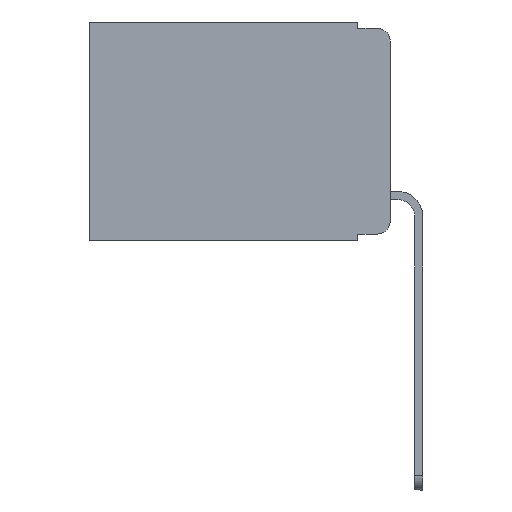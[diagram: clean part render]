
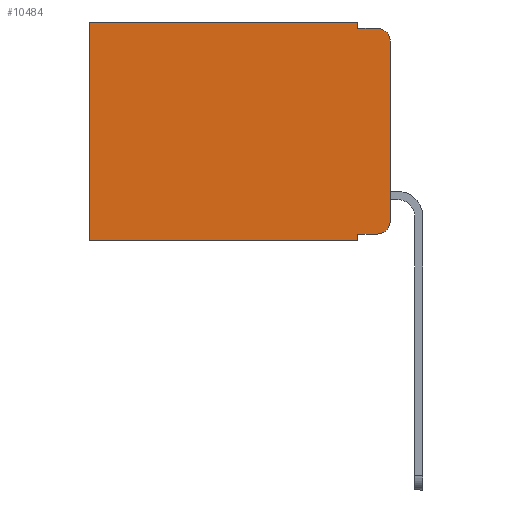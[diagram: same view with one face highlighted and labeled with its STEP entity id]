
A CAD part, left-side view. The second image highlights one B-rep face of the part: STEP entity #10484.
In plain terms, the highlighted planar face has unit normal (-1, 0, 0).
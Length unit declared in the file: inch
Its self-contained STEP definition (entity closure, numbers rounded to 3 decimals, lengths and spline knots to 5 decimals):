
#246 = CARTESIAN_POINT ( 'NONE',  ( 0.298, 0.473, 0. ) ) ;
#336 = VERTEX_POINT ( 'NONE', #1323 ) ;
#412 = DIRECTION ( 'NONE',  ( 0., 1., 0. ) ) ;
#596 = DIRECTION ( 'NONE',  ( 0., 0., -1. ) ) ;
#643 = DIRECTION ( 'NONE',  ( 0., 0., -1. ) ) ;
#776 = CARTESIAN_POINT ( 'NONE',  ( 0.298, 0., -0.343 ) ) ;
#867 = ORIENTED_EDGE ( 'NONE', *, *, #1271, .F. ) ;
#1121 = VERTEX_POINT ( 'NONE', #10203 ) ;
#1159 = ORIENTED_EDGE ( 'NONE', *, *, #6632, .T. ) ;
#1271 = EDGE_CURVE ( 'NONE', #4953, #336, #5555, .T. ) ;
#1323 = CARTESIAN_POINT ( 'NONE',  ( 0.298, 0.02, -0.01 ) ) ;
#1440 = VECTOR ( 'NONE', #6794, 39.37008 ) ;
#1689 = LINE ( 'NONE', #5073, #1440 ) ;
#2042 = EDGE_CURVE ( 'NONE', #4175, #6523, #2232, .T. ) ;
#2195 = LINE ( 'NONE', #9976, #4772 ) ;
#2226 = DIRECTION ( 'NONE',  ( -1., 0., 0. ) ) ;
#2232 = LINE ( 'NONE', #4803, #10056 ) ;
#2279 = EDGE_LOOP ( 'NONE', ( #7759, #1159, #867, #7709, #9970, #9545, #9791, #10288, #2956, #4319 ) ) ;
#2368 = CARTESIAN_POINT ( 'NONE',  ( 0.298, 0., 0. ) ) ;
#2416 = DIRECTION ( 'NONE',  ( 0., 0., -1. ) ) ;
#2614 = CARTESIAN_POINT ( 'NONE',  ( 0.298, 0., -0.03 ) ) ;
#2847 = DIRECTION ( 'NONE',  ( 0., -1., 0. ) ) ;
#2956 = ORIENTED_EDGE ( 'NONE', *, *, #5288, .T. ) ;
#3245 = CARTESIAN_POINT ( 'NONE',  ( 0.298, 0., 0. ) ) ;
#3352 = DIRECTION ( 'NONE',  ( 0., 0., -1. ) ) ;
#3495 = EDGE_CURVE ( 'NONE', #6523, #5057, #2195, .T. ) ;
#3515 = CARTESIAN_POINT ( 'NONE',  ( 0.298, 0.051, -0.333 ) ) ;
#3539 = VERTEX_POINT ( 'NONE', #5753 ) ;
#3548 = CIRCLE ( 'NONE', #7241, 0.02 ) ;
#4175 = VERTEX_POINT ( 'NONE', #5488 ) ;
#4253 = LINE ( 'NONE', #3245, #5478 ) ;
#4319 = ORIENTED_EDGE ( 'NONE', *, *, #6346, .T. ) ;
#4366 = DIRECTION ( 'NONE',  ( 0., -1., 0. ) ) ;
#4491 = VECTOR ( 'NONE', #8370, 39.37008 ) ;
#4606 = AXIS2_PLACEMENT_3D ( 'NONE', #6358, #5123, #10894 ) ;
#4772 = VECTOR ( 'NONE', #2416, 39.37008 ) ;
#4803 = CARTESIAN_POINT ( 'NONE',  ( 0.298, 0., 0. ) ) ;
#4953 = VERTEX_POINT ( 'NONE', #9632 ) ;
#5057 = VERTEX_POINT ( 'NONE', #7377 ) ;
#5073 = CARTESIAN_POINT ( 'NONE',  ( 0.298, 0.051, 0. ) ) ;
#5123 = DIRECTION ( 'NONE',  ( -1., 0., 0. ) ) ;
#5199 = CARTESIAN_POINT ( 'NONE',  ( 0.298, 0., -0.313 ) ) ;
#5288 = EDGE_CURVE ( 'NONE', #1121, #3539, #10131, .T. ) ;
#5478 = VECTOR ( 'NONE', #3352, 39.37008 ) ;
#5488 = CARTESIAN_POINT ( 'NONE',  ( 0.298, 0.051, 0. ) ) ;
#5555 = LINE ( 'NONE', #10557, #8685 ) ;
#5753 = CARTESIAN_POINT ( 'NONE',  ( 0.298, 0.02, -0.333 ) ) ;
#6346 = EDGE_CURVE ( 'NONE', #3539, #10523, #8875, .T. ) ;
#6358 = CARTESIAN_POINT ( 'NONE',  ( 0.298, 0.02, -0.313 ) ) ;
#6388 = EDGE_CURVE ( 'NONE', #7396, #10523, #4253, .T. ) ;
#6406 = CARTESIAN_POINT ( 'NONE',  ( 0.298, 0.02, -0.03 ) ) ;
#6480 = DIRECTION ( 'NONE',  ( 1., 0., 0. ) ) ;
#6523 = VERTEX_POINT ( 'NONE', #246 ) ;
#6632 = EDGE_CURVE ( 'NONE', #7396, #336, #3548, .T. ) ;
#6700 = VECTOR ( 'NONE', #4366, 39.37008 ) ;
#6794 = DIRECTION ( 'NONE',  ( 0., 0., -1. ) ) ;
#7103 = VERTEX_POINT ( 'NONE', #7247 ) ;
#7241 = AXIS2_PLACEMENT_3D ( 'NONE', #6406, #2226, #10667 ) ;
#7247 = CARTESIAN_POINT ( 'NONE',  ( 0.298, 0.051, -0.343 ) ) ;
#7377 = CARTESIAN_POINT ( 'NONE',  ( 0.298, 0.473, -0.343 ) ) ;
#7396 = VERTEX_POINT ( 'NONE', #2614 ) ;
#7709 = ORIENTED_EDGE ( 'NONE', *, *, #9335, .F. ) ;
#7759 = ORIENTED_EDGE ( 'NONE', *, *, #6388, .F. ) ;
#8154 = FACE_OUTER_BOUND ( 'NONE', #2279, .T. ) ;
#8331 = AXIS2_PLACEMENT_3D ( 'NONE', #2368, #6480, #596 ) ;
#8370 = DIRECTION ( 'NONE',  ( 0., 1., 0. ) ) ;
#8685 = VECTOR ( 'NONE', #2847, 39.37008 ) ;
#8875 = CIRCLE ( 'NONE', #4606, 0.02 ) ;
#9335 = EDGE_CURVE ( 'NONE', #4175, #4953, #10740, .T. ) ;
#9373 = LINE ( 'NONE', #776, #4491 ) ;
#9545 = ORIENTED_EDGE ( 'NONE', *, *, #3495, .T. ) ;
#9550 = EDGE_CURVE ( 'NONE', #1121, #7103, #1689, .T. ) ;
#9632 = CARTESIAN_POINT ( 'NONE',  ( 0.298, 0.051, -0.01 ) ) ;
#9791 = ORIENTED_EDGE ( 'NONE', *, *, #10602, .F. ) ;
#9970 = ORIENTED_EDGE ( 'NONE', *, *, #2042, .T. ) ;
#9976 = CARTESIAN_POINT ( 'NONE',  ( 0.298, 0.473, 0. ) ) ;
#10026 = CARTESIAN_POINT ( 'NONE',  ( 0.298, 0.051, 0. ) ) ;
#10056 = VECTOR ( 'NONE', #412, 39.37008 ) ;
#10131 = LINE ( 'NONE', #3515, #6700 ) ;
#10203 = CARTESIAN_POINT ( 'NONE',  ( 0.298, 0.051, -0.333 ) ) ;
#10288 = ORIENTED_EDGE ( 'NONE', *, *, #9550, .F. ) ;
#10484 = ADVANCED_FACE ( 'NONE', ( #8154 ), #10636, .F. ) ;
#10523 = VERTEX_POINT ( 'NONE', #5199 ) ;
#10557 = CARTESIAN_POINT ( 'NONE',  ( 0.298, 0.051, -0.01 ) ) ;
#10602 = EDGE_CURVE ( 'NONE', #7103, #5057, #9373, .T. ) ;
#10636 = PLANE ( 'NONE',  #8331 ) ;
#10667 = DIRECTION ( 'NONE',  ( 0., 0., -1. ) ) ;
#10740 = LINE ( 'NONE', #10026, #10771 ) ;
#10771 = VECTOR ( 'NONE', #643, 39.37008 ) ;
#10894 = DIRECTION ( 'NONE',  ( 0., 0., -1. ) ) ;
